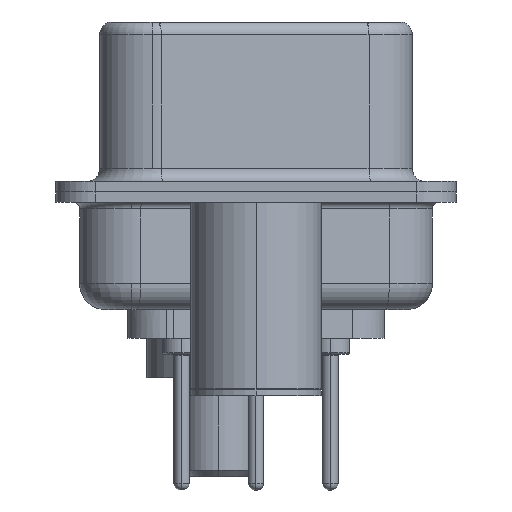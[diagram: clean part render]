
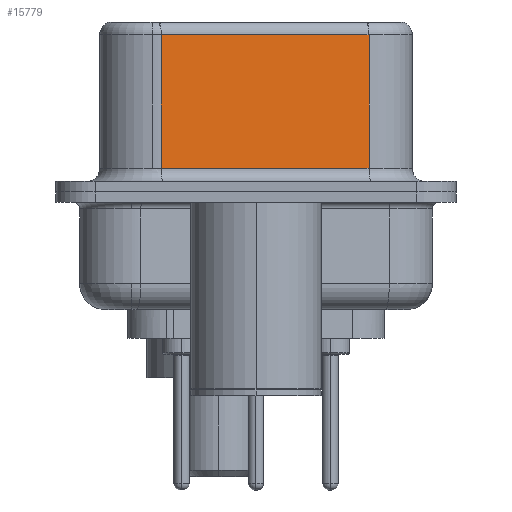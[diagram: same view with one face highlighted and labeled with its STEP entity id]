
A CAD part, left-side view. The second image highlights one B-rep face of the part: STEP entity #15779.
In plain terms, the highlighted planar face has unit normal (-0.985, -0.174, 0).
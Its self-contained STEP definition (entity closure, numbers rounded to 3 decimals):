
#1812 = VECTOR ( 'NONE', #5252, 1000. ) ;
#3004 = EDGE_LOOP ( 'NONE', ( #11456, #16978, #18931, #17552 ) ) ;
#3416 = LINE ( 'NONE', #15741, #1812 ) ;
#5252 = DIRECTION ( 'NONE',  ( 0.174, -0.985, 0. ) ) ;
#5702 = LINE ( 'NONE', #21968, #31736 ) ;
#7373 = EDGE_CURVE ( 'NONE', #18383, #32077, #5702, .T. ) ;
#9465 = CARTESIAN_POINT ( 'NONE',  ( 5.132, -4.322, 6.52 ) ) ;
#10900 = LINE ( 'NONE', #33029, #18627 ) ;
#11109 = CARTESIAN_POINT ( 'NONE',  ( 5.132, -4.322, 6.02 ) ) ;
#11456 = ORIENTED_EDGE ( 'NONE', *, *, #7373, .F. ) ;
#12567 = DIRECTION ( 'NONE',  ( -0.174, 0.985, 0. ) ) ;
#12901 = CARTESIAN_POINT ( 'NONE',  ( 3.73, 3.628, 6.52 ) ) ;
#15741 = CARTESIAN_POINT ( 'NONE',  ( 5.132, -4.322, 0.9 ) ) ;
#15779 = ADVANCED_FACE ( 'NONE', ( #22317 ), #25044, .F. ) ;
#15832 = VECTOR ( 'NONE', #20605, 1000. ) ;
#16616 = DIRECTION ( 'NONE',  ( 0., 0., -1. ) ) ;
#16706 = CARTESIAN_POINT ( 'NONE',  ( 3.73, 3.628, 6.02 ) ) ;
#16978 = ORIENTED_EDGE ( 'NONE', *, *, #16989, .T. ) ;
#16989 = EDGE_CURVE ( 'NONE', #18383, #26182, #10900, .T. ) ;
#17552 = ORIENTED_EDGE ( 'NONE', *, *, #22205, .T. ) ;
#18383 = VERTEX_POINT ( 'NONE', #11109 ) ;
#18627 = VECTOR ( 'NONE', #12567, 1000. ) ;
#18931 = ORIENTED_EDGE ( 'NONE', *, *, #32601, .T. ) ;
#20605 = DIRECTION ( 'NONE',  ( 0., 0., -1. ) ) ;
#20648 = CARTESIAN_POINT ( 'NONE',  ( 5.132, -4.322, 0.9 ) ) ;
#21968 = CARTESIAN_POINT ( 'NONE',  ( 5.132, -4.322, 6.52 ) ) ;
#22205 = EDGE_CURVE ( 'NONE', #24939, #32077, #3416, .T. ) ;
#22317 = FACE_OUTER_BOUND ( 'NONE', #3004, .T. ) ;
#24939 = VERTEX_POINT ( 'NONE', #28980 ) ;
#25044 = PLANE ( 'NONE',  #26620 ) ;
#25766 = DIRECTION ( 'NONE',  ( -0.174, 0.985, 0. ) ) ;
#26182 = VERTEX_POINT ( 'NONE', #16706 ) ;
#26620 = AXIS2_PLACEMENT_3D ( 'NONE', #9465, #27634, #25766 ) ;
#27167 = LINE ( 'NONE', #12901, #15832 ) ;
#27634 = DIRECTION ( 'NONE',  ( 0.985, 0.174, 0. ) ) ;
#28980 = CARTESIAN_POINT ( 'NONE',  ( 3.73, 3.628, 0.9 ) ) ;
#31736 = VECTOR ( 'NONE', #16616, 1000. ) ;
#32077 = VERTEX_POINT ( 'NONE', #20648 ) ;
#32601 = EDGE_CURVE ( 'NONE', #26182, #24939, #27167, .T. ) ;
#33029 = CARTESIAN_POINT ( 'NONE',  ( 5.132, -4.322, 6.02 ) ) ;
